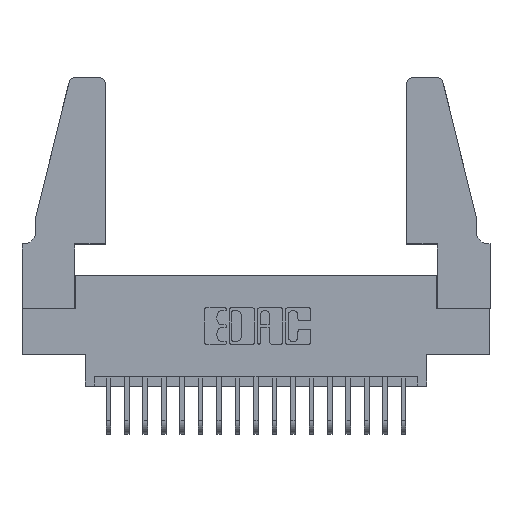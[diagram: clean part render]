
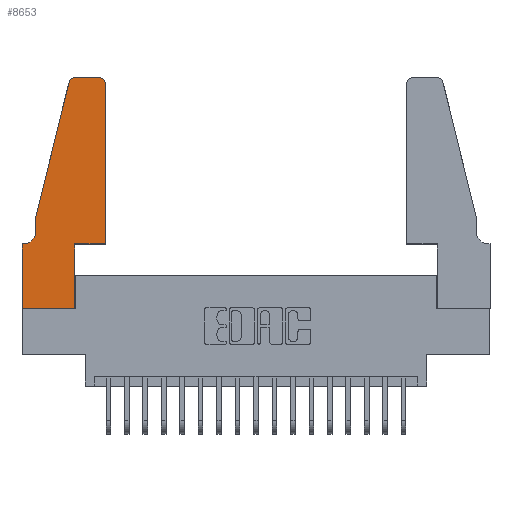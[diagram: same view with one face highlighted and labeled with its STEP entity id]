
A CAD part, top view. The second image highlights one B-rep face of the part: STEP entity #8653.
In plain terms, the highlighted planar face has unit normal (0, 0, 1).
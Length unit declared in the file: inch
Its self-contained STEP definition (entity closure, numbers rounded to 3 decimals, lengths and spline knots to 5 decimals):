
#420 = CARTESIAN_POINT ( 'NONE',  ( 0.0755, 0.5, 0.37 ) ) ;
#541 = DIRECTION ( 'NONE',  ( 1., 0., 0. ) ) ;
#1241 = CARTESIAN_POINT ( 'NONE',  ( 0.0755, 0.42, 0.37 ) ) ;
#1420 = VERTEX_POINT ( 'NONE', #19542 ) ;
#1445 = VERTEX_POINT ( 'NONE', #8618 ) ;
#1670 = CARTESIAN_POINT ( 'NONE',  ( 0.4505, 1.22, 0.37 ) ) ;
#1736 = ORIENTED_EDGE ( 'NONE', *, *, #8479, .T. ) ;
#1775 = CARTESIAN_POINT ( 'NONE',  ( 0.284, 1.25, 0.37 ) ) ;
#1911 = VECTOR ( 'NONE', #19602, 39.37008 ) ;
#2103 = DIRECTION ( 'NONE',  ( -1., 0., 0. ) ) ;
#2348 = AXIS2_PLACEMENT_3D ( 'NONE', #8729, #19909, #541 ) ;
#2375 = CARTESIAN_POINT ( 'NONE',  ( 0., 0., 0.37 ) ) ;
#2499 = CARTESIAN_POINT ( 'NONE',  ( 0.0055, 0.35, 0.37 ) ) ;
#2723 = VERTEX_POINT ( 'NONE', #15746 ) ;
#2781 = ORIENTED_EDGE ( 'NONE', *, *, #2934, .T. ) ;
#2835 = CARTESIAN_POINT ( 'NONE',  ( 0.4205, 1.22, 0.37 ) ) ;
#2917 = CARTESIAN_POINT ( 'NONE',  ( 0.4505, 0.35, 0.37 ) ) ;
#2934 = EDGE_CURVE ( 'NONE', #14038, #17724, #10533, .T. ) ;
#3135 = ORIENTED_EDGE ( 'NONE', *, *, #11698, .T. ) ;
#3148 = EDGE_CURVE ( 'NONE', #7446, #9841, #11766, .T. ) ;
#3200 = VECTOR ( 'NONE', #8748, 39.37008 ) ;
#3328 = LINE ( 'NONE', #19806, #5077 ) ;
#3645 = LINE ( 'NONE', #19934, #15107 ) ;
#3917 = CARTESIAN_POINT ( 'NONE',  ( 0., 0.35, 0.37 ) ) ;
#4465 = CIRCLE ( 'NONE', #7791, 0.03 ) ;
#5030 = CARTESIAN_POINT ( 'NONE',  ( 0.0755, 0.5, 0.37 ) ) ;
#5077 = VECTOR ( 'NONE', #5638, 39.37008 ) ;
#5083 = VERTEX_POINT ( 'NONE', #1670 ) ;
#5105 = CARTESIAN_POINT ( 'NONE',  ( 0.2865, 0.35, 0.37 ) ) ;
#5638 = DIRECTION ( 'NONE',  ( -1., 0., 0. ) ) ;
#5894 = EDGE_CURVE ( 'NONE', #5083, #2723, #4465, .T. ) ;
#5906 = CIRCLE ( 'NONE', #17952, 0.07 ) ;
#6145 = ORIENTED_EDGE ( 'NONE', *, *, #5894, .T. ) ;
#6407 = DIRECTION ( 'NONE',  ( 0., 0., -1. ) ) ;
#7446 = VERTEX_POINT ( 'NONE', #9281 ) ;
#7548 = VECTOR ( 'NONE', #15371, 39.37008 ) ;
#7791 = AXIS2_PLACEMENT_3D ( 'NONE', #2835, #15714, #8061 ) ;
#7882 = VECTOR ( 'NONE', #13429, 39.37008 ) ;
#7885 = ORIENTED_EDGE ( 'NONE', *, *, #12840, .T. ) ;
#8061 = DIRECTION ( 'NONE',  ( 1., 0., 0. ) ) ;
#8479 = EDGE_CURVE ( 'NONE', #1445, #1420, #18035, .T. ) ;
#8485 = ORIENTED_EDGE ( 'NONE', *, *, #3148, .T. ) ;
#8503 = DIRECTION ( 'NONE',  ( 0., 0., 1. ) ) ;
#8618 = CARTESIAN_POINT ( 'NONE',  ( 0., 0., 0.37 ) ) ;
#8653 = ADVANCED_FACE ( 'NONE', ( #15257 ), #14782, .T. ) ;
#8729 = CARTESIAN_POINT ( 'NONE',  ( 0.284, 1.22, 0.37 ) ) ;
#8748 = DIRECTION ( 'NONE',  ( 0., 1., 0. ) ) ;
#8824 = CARTESIAN_POINT ( 'NONE',  ( 0.4505, 0.35, 0.37 ) ) ;
#9281 = CARTESIAN_POINT ( 'NONE',  ( 0.2865, 0.35, 0.37 ) ) ;
#9841 = VERTEX_POINT ( 'NONE', #2917 ) ;
#10188 = VECTOR ( 'NONE', #11612, 39.37008 ) ;
#10286 = DIRECTION ( 'NONE',  ( -1., 0., 0. ) ) ;
#10363 = LINE ( 'NONE', #420, #1911 ) ;
#10533 = LINE ( 'NONE', #19669, #19553 ) ;
#11612 = DIRECTION ( 'NONE',  ( 0., 1., 0. ) ) ;
#11697 = CARTESIAN_POINT ( 'NONE',  ( 0.25487, 1.22718, 0.37 ) ) ;
#11698 = EDGE_CURVE ( 'NONE', #9841, #5083, #16671, .T. ) ;
#11756 = VERTEX_POINT ( 'NONE', #2499 ) ;
#11766 = LINE ( 'NONE', #8824, #7548 ) ;
#11774 = DIRECTION ( 'NONE',  ( 1., 0., 0. ) ) ;
#12683 = LINE ( 'NONE', #5105, #10188 ) ;
#12709 = EDGE_CURVE ( 'NONE', #17724, #16124, #10363, .T. ) ;
#12780 = ORIENTED_EDGE ( 'NONE', *, *, #17962, .T. ) ;
#12840 = EDGE_CURVE ( 'NONE', #17388, #1445, #16608, .T. ) ;
#13267 = VECTOR ( 'NONE', #17462, 39.37008 ) ;
#13429 = DIRECTION ( 'NONE',  ( 0., -1., 0. ) ) ;
#14038 = VERTEX_POINT ( 'NONE', #11697 ) ;
#14400 = CARTESIAN_POINT ( 'NONE',  ( 0.0055, 0.42, 0.37 ) ) ;
#14490 = EDGE_CURVE ( 'NONE', #16124, #11756, #5906, .T. ) ;
#14575 = CIRCLE ( 'NONE', #2348, 0.03 ) ;
#14782 = PLANE ( 'NONE',  #16933 ) ;
#15033 = DIRECTION ( 'NONE',  ( -0.239, -0.971, 0. ) ) ;
#15107 = VECTOR ( 'NONE', #10286, 39.37008 ) ;
#15257 = FACE_OUTER_BOUND ( 'NONE', #15412, .T. ) ;
#15360 = CARTESIAN_POINT ( 'NONE',  ( 0.4505, 0.35, 0.37 ) ) ;
#15371 = DIRECTION ( 'NONE',  ( 1., 0., 0. ) ) ;
#15412 = EDGE_LOOP ( 'NONE', ( #18441, #17661, #2781, #16076, #17692, #12780, #7885, #1736, #19687, #8485, #3135, #6145 ) ) ;
#15714 = DIRECTION ( 'NONE',  ( 0., 0., 1. ) ) ;
#15746 = CARTESIAN_POINT ( 'NONE',  ( 0.4205, 1.25, 0.37 ) ) ;
#15836 = CARTESIAN_POINT ( 'NONE',  ( 0., 0., 0.37 ) ) ;
#15981 = EDGE_CURVE ( 'NONE', #2723, #17100, #3645, .T. ) ;
#16076 = ORIENTED_EDGE ( 'NONE', *, *, #12709, .T. ) ;
#16124 = VERTEX_POINT ( 'NONE', #1241 ) ;
#16608 = LINE ( 'NONE', #2375, #7882 ) ;
#16671 = LINE ( 'NONE', #15360, #3200 ) ;
#16699 = EDGE_CURVE ( 'NONE', #17100, #14038, #14575, .T. ) ;
#16933 = AXIS2_PLACEMENT_3D ( 'NONE', #3917, #8503, #11774 ) ;
#17100 = VERTEX_POINT ( 'NONE', #1775 ) ;
#17388 = VERTEX_POINT ( 'NONE', #18343 ) ;
#17462 = DIRECTION ( 'NONE',  ( 1., 0., 0. ) ) ;
#17661 = ORIENTED_EDGE ( 'NONE', *, *, #16699, .T. ) ;
#17692 = ORIENTED_EDGE ( 'NONE', *, *, #14490, .T. ) ;
#17724 = VERTEX_POINT ( 'NONE', #5030 ) ;
#17952 = AXIS2_PLACEMENT_3D ( 'NONE', #14400, #6407, #2103 ) ;
#17962 = EDGE_CURVE ( 'NONE', #11756, #17388, #3328, .T. ) ;
#18035 = LINE ( 'NONE', #15836, #13267 ) ;
#18343 = CARTESIAN_POINT ( 'NONE',  ( 0., 0.35, 0.37 ) ) ;
#18441 = ORIENTED_EDGE ( 'NONE', *, *, #15981, .T. ) ;
#19542 = CARTESIAN_POINT ( 'NONE',  ( 0.2865, 0., 0.37 ) ) ;
#19553 = VECTOR ( 'NONE', #15033, 39.37008 ) ;
#19602 = DIRECTION ( 'NONE',  ( 0., -1., 0. ) ) ;
#19669 = CARTESIAN_POINT ( 'NONE',  ( 0.0755, 0.5, 0.37 ) ) ;
#19687 = ORIENTED_EDGE ( 'NONE', *, *, #20507, .T. ) ;
#19806 = CARTESIAN_POINT ( 'NONE',  ( 0.0755, 0.35, 0.37 ) ) ;
#19909 = DIRECTION ( 'NONE',  ( 0., 0., 1. ) ) ;
#19934 = CARTESIAN_POINT ( 'NONE',  ( 0.2605, 1.25, 0.37 ) ) ;
#20507 = EDGE_CURVE ( 'NONE', #1420, #7446, #12683, .T. ) ;
